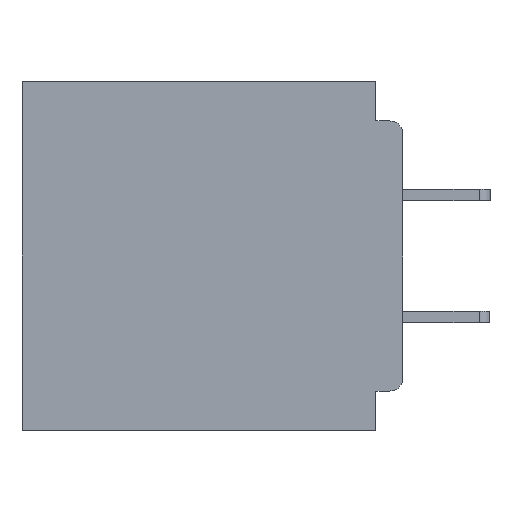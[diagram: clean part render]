
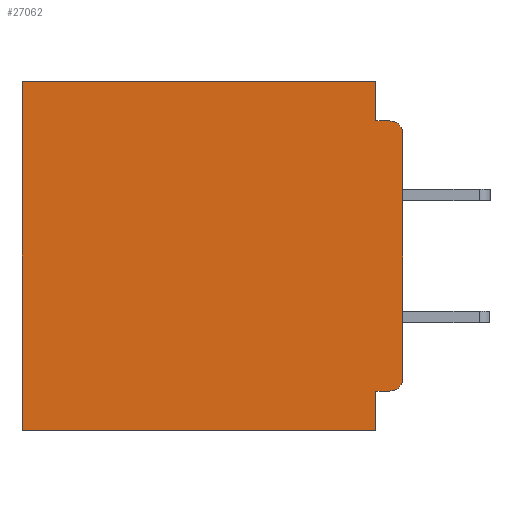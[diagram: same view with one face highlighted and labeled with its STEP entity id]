
A CAD part, left-side view. The second image highlights one B-rep face of the part: STEP entity #27062.
In plain terms, the highlighted planar face has unit normal (-1, 0, 0).
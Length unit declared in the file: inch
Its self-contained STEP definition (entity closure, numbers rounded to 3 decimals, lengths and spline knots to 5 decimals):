
#452 = ORIENTED_EDGE ( 'NONE', *, *, #22711, .F. ) ;
#1617 = CARTESIAN_POINT ( 'NONE',  ( 0.3, 0., -0.34 ) ) ;
#1639 = CARTESIAN_POINT ( 'NONE',  ( 0.3, 0.437, 0. ) ) ;
#1991 = AXIS2_PLACEMENT_3D ( 'NONE', #34784, #25510, #6585 ) ;
#2116 = ORIENTED_EDGE ( 'NONE', *, *, #24854, .F. ) ;
#3141 = VECTOR ( 'NONE', #4959, 39.37008 ) ;
#4911 = VERTEX_POINT ( 'NONE', #1617 ) ;
#4959 = DIRECTION ( 'NONE',  ( 0., 0., -1. ) ) ;
#5267 = CARTESIAN_POINT ( 'NONE',  ( 0.3, 0., -0.06 ) ) ;
#5809 = LINE ( 'NONE', #34085, #13273 ) ;
#6585 = DIRECTION ( 'NONE',  ( 0., 0., -1. ) ) ;
#7297 = CARTESIAN_POINT ( 'NONE',  ( 0.3, 0., -0.045 ) ) ;
#8623 = EDGE_CURVE ( 'NONE', #15389, #14104, #29467, .T. ) ;
#8720 = ORIENTED_EDGE ( 'NONE', *, *, #32702, .T. ) ;
#10187 = VERTEX_POINT ( 'NONE', #20989 ) ;
#10565 = CARTESIAN_POINT ( 'NONE',  ( 0.3, 0.015, -0.045 ) ) ;
#10649 = EDGE_CURVE ( 'NONE', #23869, #36326, #31758, .T. ) ;
#11217 = CARTESIAN_POINT ( 'NONE',  ( 0.3, 0.031, -0.4 ) ) ;
#11431 = CARTESIAN_POINT ( 'NONE',  ( 0.3, 0.437, -0.4 ) ) ;
#11733 = ORIENTED_EDGE ( 'NONE', *, *, #16544, .T. ) ;
#12328 = CARTESIAN_POINT ( 'NONE',  ( 0.3, 0.031, -0.4 ) ) ;
#12483 = CARTESIAN_POINT ( 'NONE',  ( 0.3, 0., 0. ) ) ;
#13273 = VECTOR ( 'NONE', #15410, 39.37008 ) ;
#13675 = CIRCLE ( 'NONE', #36411, 0.015 ) ;
#13831 = VERTEX_POINT ( 'NONE', #25430 ) ;
#14093 = VERTEX_POINT ( 'NONE', #1639 ) ;
#14104 = VERTEX_POINT ( 'NONE', #11217 ) ;
#14119 = VECTOR ( 'NONE', #17260, 39.37008 ) ;
#14993 = VECTOR ( 'NONE', #38831, 39.37008 ) ;
#15092 = EDGE_CURVE ( 'NONE', #14104, #16454, #16232, .T. ) ;
#15111 = DIRECTION ( 'NONE',  ( -1., 0., 0. ) ) ;
#15389 = VERTEX_POINT ( 'NONE', #24603 ) ;
#15410 = DIRECTION ( 'NONE',  ( 0., 0., -1. ) ) ;
#15467 = DIRECTION ( 'NONE',  ( -1., 0., 0. ) ) ;
#15734 = DIRECTION ( 'NONE',  ( 0., 1., 0. ) ) ;
#16232 = LINE ( 'NONE', #20183, #40739 ) ;
#16454 = VERTEX_POINT ( 'NONE', #11431 ) ;
#16544 = EDGE_CURVE ( 'NONE', #10187, #4911, #37207, .T. ) ;
#16746 = ORIENTED_EDGE ( 'NONE', *, *, #15092, .F. ) ;
#17260 = DIRECTION ( 'NONE',  ( 0., 0., -1. ) ) ;
#18733 = EDGE_CURVE ( 'NONE', #13831, #14093, #20823, .T. ) ;
#20183 = CARTESIAN_POINT ( 'NONE',  ( 0.3, 0., -0.4 ) ) ;
#20477 = VECTOR ( 'NONE', #15734, 39.37008 ) ;
#20821 = ORIENTED_EDGE ( 'NONE', *, *, #18733, .T. ) ;
#20823 = LINE ( 'NONE', #12483, #31222 ) ;
#20989 = CARTESIAN_POINT ( 'NONE',  ( 0.3, 0.015, -0.355 ) ) ;
#21296 = EDGE_CURVE ( 'NONE', #13831, #23869, #5809, .T. ) ;
#22492 = LINE ( 'NONE', #32817, #14119 ) ;
#22711 = EDGE_CURVE ( 'NONE', #10187, #15389, #29895, .T. ) ;
#23385 = DIRECTION ( 'NONE',  ( 0., 1., 0. ) ) ;
#23753 = VERTEX_POINT ( 'NONE', #5267 ) ;
#23869 = VERTEX_POINT ( 'NONE', #34713 ) ;
#24121 = EDGE_CURVE ( 'NONE', #14093, #16454, #22492, .T. ) ;
#24603 = CARTESIAN_POINT ( 'NONE',  ( 0.3, 0.031, -0.355 ) ) ;
#24854 = EDGE_CURVE ( 'NONE', #23753, #4911, #28336, .T. ) ;
#25430 = CARTESIAN_POINT ( 'NONE',  ( 0.3, 0.031, 0. ) ) ;
#25510 = DIRECTION ( 'NONE',  ( 1., 0., 0. ) ) ;
#27062 = ADVANCED_FACE ( 'NONE', ( #29155 ), #37966, .F. ) ;
#28336 = LINE ( 'NONE', #33197, #3141 ) ;
#29155 = FACE_OUTER_BOUND ( 'NONE', #36598, .T. ) ;
#29467 = LINE ( 'NONE', #12328, #36753 ) ;
#29895 = LINE ( 'NONE', #37678, #20477 ) ;
#31081 = ORIENTED_EDGE ( 'NONE', *, *, #24121, .T. ) ;
#31222 = VECTOR ( 'NONE', #34407, 39.37008 ) ;
#31290 = DIRECTION ( 'NONE',  ( 0., 0., -1. ) ) ;
#31699 = AXIS2_PLACEMENT_3D ( 'NONE', #33945, #15111, #37061 ) ;
#31758 = LINE ( 'NONE', #7297, #14993 ) ;
#32702 = EDGE_CURVE ( 'NONE', #23753, #36326, #13675, .T. ) ;
#32817 = CARTESIAN_POINT ( 'NONE',  ( 0.3, 0.437, -0.4 ) ) ;
#33197 = CARTESIAN_POINT ( 'NONE',  ( 0.3, 0., -0.4 ) ) ;
#33419 = ORIENTED_EDGE ( 'NONE', *, *, #21296, .F. ) ;
#33945 = CARTESIAN_POINT ( 'NONE',  ( 0.3, 0.015, -0.34 ) ) ;
#34085 = CARTESIAN_POINT ( 'NONE',  ( 0.3, 0.031, 0. ) ) ;
#34267 = CARTESIAN_POINT ( 'NONE',  ( 0.3, 0.015, -0.06 ) ) ;
#34390 = ORIENTED_EDGE ( 'NONE', *, *, #8623, .F. ) ;
#34407 = DIRECTION ( 'NONE',  ( 0., 1., 0. ) ) ;
#34713 = CARTESIAN_POINT ( 'NONE',  ( 0.3, 0.031, -0.045 ) ) ;
#34784 = CARTESIAN_POINT ( 'NONE',  ( 0.3, 0., -0.4 ) ) ;
#36326 = VERTEX_POINT ( 'NONE', #10565 ) ;
#36411 = AXIS2_PLACEMENT_3D ( 'NONE', #34267, #15467, #37416 ) ;
#36598 = EDGE_LOOP ( 'NONE', ( #2116, #8720, #37661, #33419, #20821, #31081, #16746, #34390, #452, #11733 ) ) ;
#36753 = VECTOR ( 'NONE', #31290, 39.37008 ) ;
#37061 = DIRECTION ( 'NONE',  ( 0., 0., -1. ) ) ;
#37207 = CIRCLE ( 'NONE', #31699, 0.015 ) ;
#37416 = DIRECTION ( 'NONE',  ( 0., 0., -1. ) ) ;
#37661 = ORIENTED_EDGE ( 'NONE', *, *, #10649, .F. ) ;
#37678 = CARTESIAN_POINT ( 'NONE',  ( 0.3, 0., -0.355 ) ) ;
#37966 = PLANE ( 'NONE',  #1991 ) ;
#38831 = DIRECTION ( 'NONE',  ( 0., -1., 0. ) ) ;
#40739 = VECTOR ( 'NONE', #23385, 39.37008 ) ;
